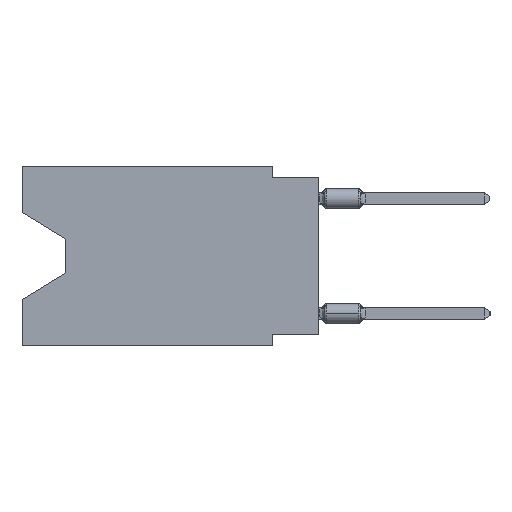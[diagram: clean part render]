
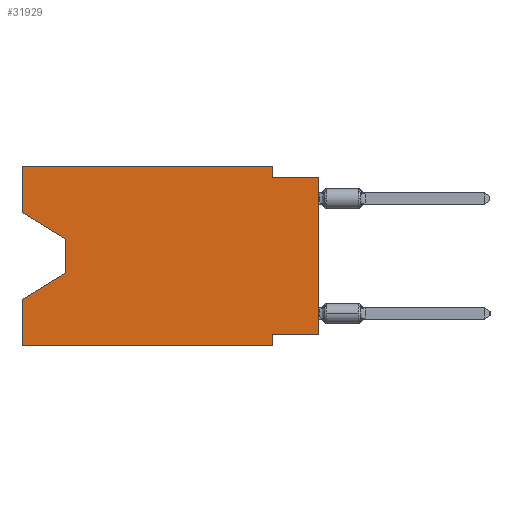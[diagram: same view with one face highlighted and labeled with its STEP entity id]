
A CAD part, left-side view. The second image highlights one B-rep face of the part: STEP entity #31929.
In plain terms, the highlighted planar face has unit normal (-1, 0, 0).
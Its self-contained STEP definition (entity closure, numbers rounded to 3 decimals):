
#329 = DIRECTION ( 'NONE',  ( 0., 0., 1. ) ) ;
#349 = ORIENTED_EDGE ( 'NONE', *, *, #37193, .F. ) ;
#518 = DIRECTION ( 'NONE',  ( 0., 0., -1. ) ) ;
#592 = VECTOR ( 'NONE', #518, 1000. ) ;
#1354 = ORIENTED_EDGE ( 'NONE', *, *, #17822, .T. ) ;
#1562 = CARTESIAN_POINT ( 'NONE',  ( 0., 16.383, -9.906 ) ) ;
#1591 = LINE ( 'NONE', #15948, #42804 ) ;
#2176 = EDGE_CURVE ( 'NONE', #6325, #27777, #1591, .T. ) ;
#2298 = CARTESIAN_POINT ( 'NONE',  ( 0., 2.54, -9.906 ) ) ;
#4213 = CARTESIAN_POINT ( 'NONE',  ( 0., 16.383, 0. ) ) ;
#5813 = LINE ( 'NONE', #13813, #43098 ) ;
#5855 = ORIENTED_EDGE ( 'NONE', *, *, #31837, .T. ) ;
#6068 = CARTESIAN_POINT ( 'NONE',  ( 0., 16.383, -7.36 ) ) ;
#6183 = VECTOR ( 'NONE', #32119, 1000. ) ;
#6325 = VERTEX_POINT ( 'NONE', #29266 ) ;
#6698 = VECTOR ( 'NONE', #36300, 1000. ) ;
#7977 = CARTESIAN_POINT ( 'NONE',  ( 0., 16.383, 0. ) ) ;
#8577 = LINE ( 'NONE', #30722, #37645 ) ;
#8734 = VERTEX_POINT ( 'NONE', #22203 ) ;
#8748 = EDGE_CURVE ( 'NONE', #34460, #42623, #25500, .T. ) ;
#8790 = CARTESIAN_POINT ( 'NONE',  ( 0., 16.383, -9.906 ) ) ;
#10050 = DIRECTION ( 'NONE',  ( 0., 0., 1. ) ) ;
#10615 = VECTOR ( 'NONE', #329, 1000. ) ;
#10967 = VECTOR ( 'NONE', #25916, 1000. ) ;
#11222 = LINE ( 'NONE', #39775, #19885 ) ;
#11834 = LINE ( 'NONE', #26242, #10615 ) ;
#11985 = EDGE_CURVE ( 'NONE', #27777, #8734, #29057, .T. ) ;
#12211 = LINE ( 'NONE', #43849, #10967 ) ;
#12372 = DIRECTION ( 'NONE',  ( 0., -1., 0. ) ) ;
#13086 = VERTEX_POINT ( 'NONE', #17689 ) ;
#13801 = CARTESIAN_POINT ( 'NONE',  ( 0., 0., 0. ) ) ;
#13813 = CARTESIAN_POINT ( 'NONE',  ( 0., 16.383, 0. ) ) ;
#13854 = CARTESIAN_POINT ( 'NONE',  ( 0., 13.97, -4.013 ) ) ;
#13977 = EDGE_CURVE ( 'NONE', #16158, #6325, #5813, .T. ) ;
#15053 = DIRECTION ( 'NONE',  ( 1., 0., 0. ) ) ;
#15230 = VECTOR ( 'NONE', #16646, 1000. ) ;
#15393 = DIRECTION ( 'NONE',  ( 0., 1., 0. ) ) ;
#15539 = VECTOR ( 'NONE', #12372, 1000. ) ;
#15948 = CARTESIAN_POINT ( 'NONE',  ( 0., 2.54, 0. ) ) ;
#16158 = VERTEX_POINT ( 'NONE', #39210 ) ;
#16559 = EDGE_CURVE ( 'NONE', #42623, #17610, #11222, .T. ) ;
#16646 = DIRECTION ( 'NONE',  ( 0., 0., -1. ) ) ;
#17444 = ORIENTED_EDGE ( 'NONE', *, *, #16559, .T. ) ;
#17610 = VERTEX_POINT ( 'NONE', #6068 ) ;
#17689 = CARTESIAN_POINT ( 'NONE',  ( 0., 16.383, -2.546 ) ) ;
#17822 = EDGE_CURVE ( 'NONE', #40013, #35436, #19438, .T. ) ;
#19438 = LINE ( 'NONE', #1562, #15539 ) ;
#19885 = VECTOR ( 'NONE', #25623, 1000. ) ;
#22093 = ORIENTED_EDGE ( 'NONE', *, *, #39116, .F. ) ;
#22203 = CARTESIAN_POINT ( 'NONE',  ( 0., 0., -0.635 ) ) ;
#22206 = VERTEX_POINT ( 'NONE', #22219 ) ;
#22219 = CARTESIAN_POINT ( 'NONE',  ( 0., 2.54, -9.271 ) ) ;
#22251 = ORIENTED_EDGE ( 'NONE', *, *, #29304, .F. ) ;
#22357 = LINE ( 'NONE', #7977, #6698 ) ;
#22359 = PLANE ( 'NONE',  #38160 ) ;
#22911 = ORIENTED_EDGE ( 'NONE', *, *, #8748, .T. ) ;
#23882 = ORIENTED_EDGE ( 'NONE', *, *, #34780, .T. ) ;
#24180 = ORIENTED_EDGE ( 'NONE', *, *, #13977, .F. ) ;
#25500 = LINE ( 'NONE', #25978, #592 ) ;
#25623 = DIRECTION ( 'NONE',  ( 0., 0.855, -0.519 ) ) ;
#25713 = CARTESIAN_POINT ( 'NONE',  ( 0., 2.54, -0.635 ) ) ;
#25916 = DIRECTION ( 'NONE',  ( 0., -0.855, -0.519 ) ) ;
#25978 = CARTESIAN_POINT ( 'NONE',  ( 0., 13.97, -4.013 ) ) ;
#26242 = CARTESIAN_POINT ( 'NONE',  ( 0., 16.383, 0. ) ) ;
#27777 = VERTEX_POINT ( 'NONE', #25713 ) ;
#28533 = VECTOR ( 'NONE', #10050, 1000. ) ;
#29057 = LINE ( 'NONE', #38755, #6183 ) ;
#29266 = CARTESIAN_POINT ( 'NONE',  ( 0., 2.54, 0. ) ) ;
#29304 = EDGE_CURVE ( 'NONE', #22206, #35436, #34585, .T. ) ;
#29322 = CARTESIAN_POINT ( 'NONE',  ( 0., 2.54, -9.906 ) ) ;
#29464 = DIRECTION ( 'NONE',  ( 0., 0., -1. ) ) ;
#30357 = DIRECTION ( 'NONE',  ( 0., 0., -1. ) ) ;
#30722 = CARTESIAN_POINT ( 'NONE',  ( 0., 0., -9.271 ) ) ;
#31837 = EDGE_CURVE ( 'NONE', #13086, #34460, #12211, .T. ) ;
#31929 = ADVANCED_FACE ( 'NONE', ( #36521 ), #22359, .F. ) ;
#32019 = VERTEX_POINT ( 'NONE', #38387 ) ;
#32119 = DIRECTION ( 'NONE',  ( 0., -1., 0. ) ) ;
#32180 = ORIENTED_EDGE ( 'NONE', *, *, #11985, .F. ) ;
#34197 = ORIENTED_EDGE ( 'NONE', *, *, #2176, .F. ) ;
#34460 = VERTEX_POINT ( 'NONE', #13854 ) ;
#34585 = LINE ( 'NONE', #2298, #15230 ) ;
#34780 = EDGE_CURVE ( 'NONE', #32019, #8734, #45895, .T. ) ;
#35436 = VERTEX_POINT ( 'NONE', #29322 ) ;
#36184 = EDGE_LOOP ( 'NONE', ( #5855, #22911, #17444, #349, #1354, #22251, #39590, #23882, #32180, #34197, #24180, #22093 ) ) ;
#36300 = DIRECTION ( 'NONE',  ( 0., 0., 1. ) ) ;
#36521 = FACE_OUTER_BOUND ( 'NONE', #36184, .T. ) ;
#37193 = EDGE_CURVE ( 'NONE', #40013, #17610, #11834, .T. ) ;
#37645 = VECTOR ( 'NONE', #15393, 1000. ) ;
#38160 = AXIS2_PLACEMENT_3D ( 'NONE', #4213, #15053, #29464 ) ;
#38387 = CARTESIAN_POINT ( 'NONE',  ( 0., 0., -9.271 ) ) ;
#38755 = CARTESIAN_POINT ( 'NONE',  ( 0., 0., -0.635 ) ) ;
#39116 = EDGE_CURVE ( 'NONE', #13086, #16158, #22357, .T. ) ;
#39210 = CARTESIAN_POINT ( 'NONE',  ( 0., 16.383, 0. ) ) ;
#39590 = ORIENTED_EDGE ( 'NONE', *, *, #40037, .F. ) ;
#39775 = CARTESIAN_POINT ( 'NONE',  ( 0., 13.97, -5.893 ) ) ;
#40013 = VERTEX_POINT ( 'NONE', #8790 ) ;
#40037 = EDGE_CURVE ( 'NONE', #32019, #22206, #8577, .T. ) ;
#42623 = VERTEX_POINT ( 'NONE', #44148 ) ;
#42804 = VECTOR ( 'NONE', #30357, 1000. ) ;
#43098 = VECTOR ( 'NONE', #45660, 1000. ) ;
#43849 = CARTESIAN_POINT ( 'NONE',  ( 0., 16.383, -2.546 ) ) ;
#44148 = CARTESIAN_POINT ( 'NONE',  ( 0., 13.97, -5.893 ) ) ;
#45660 = DIRECTION ( 'NONE',  ( 0., -1., 0. ) ) ;
#45895 = LINE ( 'NONE', #13801, #28533 ) ;
